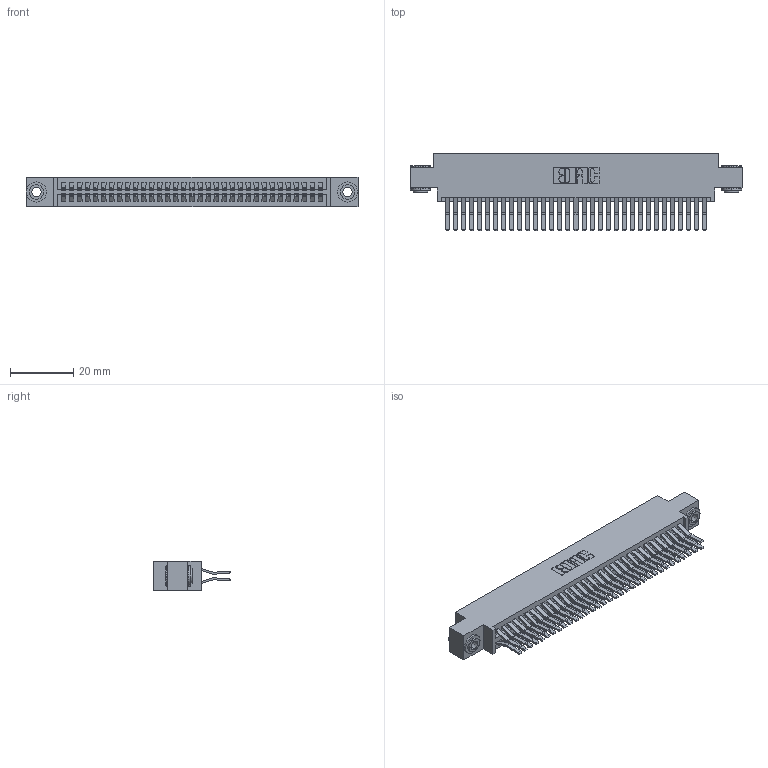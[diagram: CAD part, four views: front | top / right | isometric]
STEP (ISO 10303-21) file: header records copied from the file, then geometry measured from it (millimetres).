
FILE_DESCRIPTION (( 'STEP AP203' ), '1' );
FILE_NAME ('345-066-560-803.STEP', '2019-10-30T18:59:12', ( '' ), ( '' ), 'SwSTEP 2.0', 'SolidWorks 2016', '' );
FILE_SCHEMA (( 'CONFIG_CONTROL_DESIGN' ));
Length unit declared in the file: inch
Products named in the file (4): 345-066-560-803; 345-292-001_560 Tail; 345 Part_0.170 Offset - 0.156 Dia-TH; 345-250-002_345-250-002-102
Assembly tree (69 placements, depth 2):
  345-066-560-803
    345 Part_0.170 Offset - 0.156 Dia-TH
    345-292-001_560 Tail  x66
    345-250-002_345-250-002-102  x2
Bounding box: 105.03 x 24.45 x 9.4 mm (x, y, z)
Volume: 10457.7 mm3; surface area: 16744.9 mm2
Topology: 69 solids, 69 shells, 3600 faces, 10659 edges, 7014 vertices
Faces by surface type: plane 2272, cylinder 1320, cone 8
Entity records: 27974 total; most frequent: CARTESIAN_POINT 4675, ORIENTED_EDGE 4602, DIRECTION 4167, EDGE_CURVE 2301, VECTOR 2009, LINE 2009, VERTEX_POINT 1530, AXIS2_PLACEMENT_3D 1079
